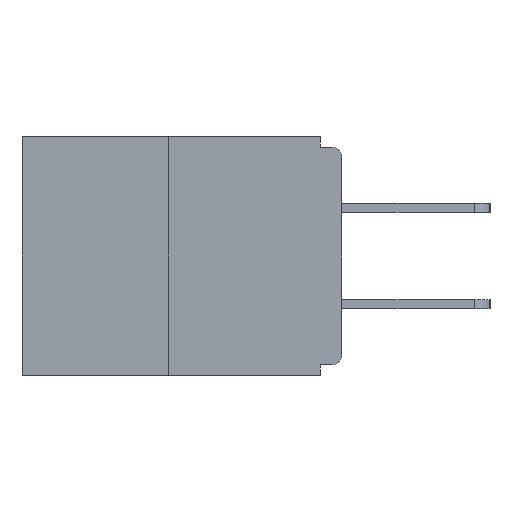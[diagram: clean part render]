
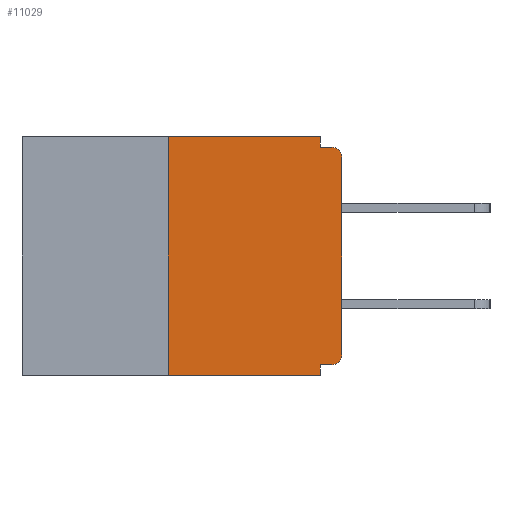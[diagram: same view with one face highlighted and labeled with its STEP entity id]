
A CAD part, left-side view. The second image highlights one B-rep face of the part: STEP entity #11029.
In plain terms, the highlighted planar face has unit normal (-1, 0, 0).
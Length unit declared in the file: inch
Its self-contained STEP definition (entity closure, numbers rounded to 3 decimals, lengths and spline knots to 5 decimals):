
#330 = PLANE ( 'NONE',  #30197 ) ;
#750 = ORIENTED_EDGE ( 'NONE', *, *, #6645, .F. ) ;
#1162 = VECTOR ( 'NONE', #5411, 39.37008 ) ;
#1388 = ORIENTED_EDGE ( 'NONE', *, *, #6630, .T. ) ;
#1433 = FACE_OUTER_BOUND ( 'NONE', #14351, .T. ) ;
#2443 = CARTESIAN_POINT ( 'NONE',  ( 0., 0., 0. ) ) ;
#2950 = CARTESIAN_POINT ( 'NONE',  ( 0., 0.46, 0. ) ) ;
#3202 = VERTEX_POINT ( 'NONE', #20967 ) ;
#3420 = DIRECTION ( 'NONE',  ( 0., -1., 0. ) ) ;
#3485 = CARTESIAN_POINT ( 'NONE',  ( 0., 0.031, -0.343 ) ) ;
#3599 = ORIENTED_EDGE ( 'NONE', *, *, #9880, .F. ) ;
#4191 = EDGE_CURVE ( 'NONE', #13220, #9687, #19987, .T. ) ;
#4408 = ORIENTED_EDGE ( 'NONE', *, *, #17901, .T. ) ;
#4593 = EDGE_CURVE ( 'NONE', #21884, #26823, #12552, .T. ) ;
#5303 = LINE ( 'NONE', #28349, #7836 ) ;
#5411 = DIRECTION ( 'NONE',  ( 0., 0., -1. ) ) ;
#5441 = VERTEX_POINT ( 'NONE', #6848 ) ;
#5760 = CARTESIAN_POINT ( 'NONE',  ( 0., 0., -0.313 ) ) ;
#6104 = ORIENTED_EDGE ( 'NONE', *, *, #4191, .T. ) ;
#6165 = EDGE_CURVE ( 'NONE', #12767, #27110, #17538, .T. ) ;
#6314 = LINE ( 'NONE', #31537, #19091 ) ;
#6630 = EDGE_CURVE ( 'NONE', #5441, #12767, #12794, .T. ) ;
#6645 = EDGE_CURVE ( 'NONE', #29229, #9687, #24486, .T. ) ;
#6848 = CARTESIAN_POINT ( 'NONE',  ( 0., 0.015, -0.328 ) ) ;
#7357 = VERTEX_POINT ( 'NONE', #24039 ) ;
#7836 = VECTOR ( 'NONE', #3420, 39.37008 ) ;
#8362 = DIRECTION ( 'NONE',  ( 0., 1., 0. ) ) ;
#9687 = VERTEX_POINT ( 'NONE', #3485 ) ;
#9745 = DIRECTION ( 'NONE',  ( 0., 0., 1. ) ) ;
#9880 = EDGE_CURVE ( 'NONE', #5441, #29229, #13398, .T. ) ;
#10256 = VECTOR ( 'NONE', #26504, 39.37008 ) ;
#10292 = EDGE_CURVE ( 'NONE', #7357, #3202, #5303, .T. ) ;
#10356 = DIRECTION ( 'NONE',  ( 0., 0., -1. ) ) ;
#10409 = CARTESIAN_POINT ( 'NONE',  ( 0., 0.031, -0.343 ) ) ;
#10953 = CARTESIAN_POINT ( 'NONE',  ( 0., 0.25, 0. ) ) ;
#11029 = ADVANCED_FACE ( 'NONE', ( #1433 ), #330, .F. ) ;
#11426 = DIRECTION ( 'NONE',  ( 0., 0., -1. ) ) ;
#11732 = DIRECTION ( 'NONE',  ( 0., 0., -1. ) ) ;
#12074 = CARTESIAN_POINT ( 'NONE',  ( 0., 0., -0.015 ) ) ;
#12552 = LINE ( 'NONE', #12074, #10256 ) ;
#12607 = VECTOR ( 'NONE', #8362, 39.37008 ) ;
#12767 = VERTEX_POINT ( 'NONE', #5760 ) ;
#12794 = CIRCLE ( 'NONE', #19606, 0.015 ) ;
#12830 = VECTOR ( 'NONE', #29409, 39.37008 ) ;
#12924 = CIRCLE ( 'NONE', #17593, 0.015 ) ;
#13220 = VERTEX_POINT ( 'NONE', #19797 ) ;
#13398 = LINE ( 'NONE', #20707, #12607 ) ;
#13509 = CARTESIAN_POINT ( 'NONE',  ( 0., 0.46, -0.343 ) ) ;
#13774 = CARTESIAN_POINT ( 'NONE',  ( 0., 0.031, -0.328 ) ) ;
#14351 = EDGE_LOOP ( 'NONE', ( #22985, #28957, #6104, #750, #3599, #1388, #24190, #4408, #24168, #29344 ) ) ;
#16523 = CARTESIAN_POINT ( 'NONE',  ( 0., 0.031, -0.015 ) ) ;
#16714 = DIRECTION ( 'NONE',  ( -1., 0., 0. ) ) ;
#17538 = LINE ( 'NONE', #2443, #12830 ) ;
#17593 = AXIS2_PLACEMENT_3D ( 'NONE', #21587, #16714, #11732 ) ;
#17901 = EDGE_CURVE ( 'NONE', #27110, #26823, #12924, .T. ) ;
#19091 = VECTOR ( 'NONE', #11426, 39.37008 ) ;
#19606 = AXIS2_PLACEMENT_3D ( 'NONE', #20269, #30304, #27820 ) ;
#19797 = CARTESIAN_POINT ( 'NONE',  ( 0., 0.25, -0.343 ) ) ;
#19987 = LINE ( 'NONE', #13509, #31588 ) ;
#20220 = DIRECTION ( 'NONE',  ( 1., 0., 0. ) ) ;
#20269 = CARTESIAN_POINT ( 'NONE',  ( 0., 0.015, -0.313 ) ) ;
#20707 = CARTESIAN_POINT ( 'NONE',  ( 0., 0., -0.328 ) ) ;
#20967 = CARTESIAN_POINT ( 'NONE',  ( 0., 0.031, 0. ) ) ;
#21587 = CARTESIAN_POINT ( 'NONE',  ( 0., 0.015, -0.03 ) ) ;
#21884 = VERTEX_POINT ( 'NONE', #16523 ) ;
#22899 = LINE ( 'NONE', #10953, #26766 ) ;
#22985 = ORIENTED_EDGE ( 'NONE', *, *, #10292, .F. ) ;
#23498 = CARTESIAN_POINT ( 'NONE',  ( 0., 0.015, -0.015 ) ) ;
#24039 = CARTESIAN_POINT ( 'NONE',  ( 0., 0.25, 0. ) ) ;
#24168 = ORIENTED_EDGE ( 'NONE', *, *, #4593, .F. ) ;
#24190 = ORIENTED_EDGE ( 'NONE', *, *, #6165, .T. ) ;
#24486 = LINE ( 'NONE', #10409, #1162 ) ;
#25490 = CARTESIAN_POINT ( 'NONE',  ( 0., 0., -0.03 ) ) ;
#26504 = DIRECTION ( 'NONE',  ( 0., -1., 0. ) ) ;
#26766 = VECTOR ( 'NONE', #9745, 39.37008 ) ;
#26823 = VERTEX_POINT ( 'NONE', #23498 ) ;
#27110 = VERTEX_POINT ( 'NONE', #25490 ) ;
#27820 = DIRECTION ( 'NONE',  ( 0., 0., -1. ) ) ;
#28349 = CARTESIAN_POINT ( 'NONE',  ( 0., 0.46, 0. ) ) ;
#28957 = ORIENTED_EDGE ( 'NONE', *, *, #30524, .F. ) ;
#29229 = VERTEX_POINT ( 'NONE', #13774 ) ;
#29283 = EDGE_CURVE ( 'NONE', #3202, #21884, #6314, .T. ) ;
#29344 = ORIENTED_EDGE ( 'NONE', *, *, #29283, .F. ) ;
#29409 = DIRECTION ( 'NONE',  ( 0., 0., 1. ) ) ;
#30197 = AXIS2_PLACEMENT_3D ( 'NONE', #2950, #20220, #10356 ) ;
#30304 = DIRECTION ( 'NONE',  ( -1., 0., 0. ) ) ;
#30524 = EDGE_CURVE ( 'NONE', #13220, #7357, #22899, .T. ) ;
#30941 = DIRECTION ( 'NONE',  ( 0., -1., 0. ) ) ;
#31537 = CARTESIAN_POINT ( 'NONE',  ( 0., 0.031, 0. ) ) ;
#31588 = VECTOR ( 'NONE', #30941, 39.37008 ) ;
